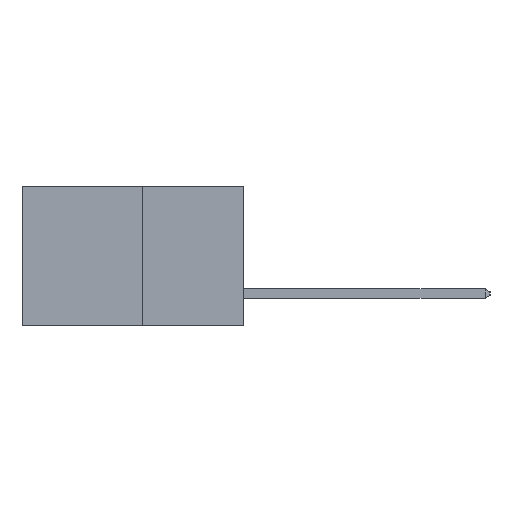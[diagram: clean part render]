
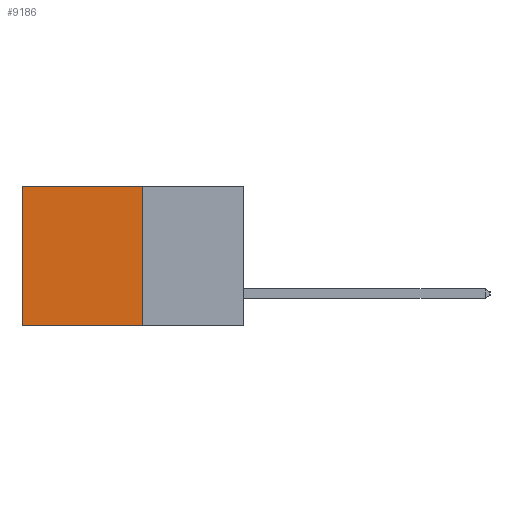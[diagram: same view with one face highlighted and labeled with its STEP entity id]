
A CAD part, left-side view. The second image highlights one B-rep face of the part: STEP entity #9186.
In plain terms, the highlighted planar face has unit normal (-1, 0, 0).
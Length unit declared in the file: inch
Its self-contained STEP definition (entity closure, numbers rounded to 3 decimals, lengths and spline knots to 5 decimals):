
#305 = VERTEX_POINT ( 'NONE', #18248 ) ;
#1296 = EDGE_CURVE ( 'NONE', #305, #4624, #8270, .T. ) ;
#1407 = CARTESIAN_POINT ( 'NONE',  ( 0.277, 0.59, 0. ) ) ;
#1757 = CARTESIAN_POINT ( 'NONE',  ( 0.277, 0.27, -0.37 ) ) ;
#2192 = VERTEX_POINT ( 'NONE', #10133 ) ;
#2246 = LINE ( 'NONE', #13829, #7796 ) ;
#2468 = ORIENTED_EDGE ( 'NONE', *, *, #18503, .F. ) ;
#3327 = VECTOR ( 'NONE', #10431, 39.37008 ) ;
#4147 = PLANE ( 'NONE',  #10761 ) ;
#4608 = EDGE_CURVE ( 'NONE', #4624, #13963, #8369, .T. ) ;
#4624 = VERTEX_POINT ( 'NONE', #1407 ) ;
#4732 = VECTOR ( 'NONE', #11727, 39.37008 ) ;
#5389 = FACE_OUTER_BOUND ( 'NONE', #13304, .T. ) ;
#6354 = CARTESIAN_POINT ( 'NONE',  ( 0.277, 0.59, -0.37 ) ) ;
#7559 = DIRECTION ( 'NONE',  ( 1., 0., 0. ) ) ;
#7796 = VECTOR ( 'NONE', #18578, 39.37008 ) ;
#8166 = LINE ( 'NONE', #1757, #4732 ) ;
#8270 = LINE ( 'NONE', #13934, #20627 ) ;
#8369 = LINE ( 'NONE', #6354, #3327 ) ;
#9186 = ADVANCED_FACE ( 'NONE', ( #5389 ), #4147, .F. ) ;
#10133 = CARTESIAN_POINT ( 'NONE',  ( 0.277, 0.27, -0.37 ) ) ;
#10417 = CARTESIAN_POINT ( 'NONE',  ( 0.277, 0.59, -0.37 ) ) ;
#10431 = DIRECTION ( 'NONE',  ( 0., 0., -1. ) ) ;
#10761 = AXIS2_PLACEMENT_3D ( 'NONE', #17292, #7559, #18899 ) ;
#11453 = ORIENTED_EDGE ( 'NONE', *, *, #13149, .F. ) ;
#11621 = ORIENTED_EDGE ( 'NONE', *, *, #1296, .T. ) ;
#11727 = DIRECTION ( 'NONE',  ( 0., 1., 0. ) ) ;
#11925 = DIRECTION ( 'NONE',  ( 0., 1., 0. ) ) ;
#13149 = EDGE_CURVE ( 'NONE', #2192, #13963, #8166, .T. ) ;
#13304 = EDGE_LOOP ( 'NONE', ( #17379, #11453, #2468, #11621 ) ) ;
#13829 = CARTESIAN_POINT ( 'NONE',  ( 0.277, 0.27, -0.37 ) ) ;
#13934 = CARTESIAN_POINT ( 'NONE',  ( 0.277, 0.27, 0. ) ) ;
#13963 = VERTEX_POINT ( 'NONE', #10417 ) ;
#17292 = CARTESIAN_POINT ( 'NONE',  ( 0.277, 0.27, -0.37 ) ) ;
#17379 = ORIENTED_EDGE ( 'NONE', *, *, #4608, .T. ) ;
#18248 = CARTESIAN_POINT ( 'NONE',  ( 0.277, 0.27, 0. ) ) ;
#18503 = EDGE_CURVE ( 'NONE', #305, #2192, #2246, .T. ) ;
#18578 = DIRECTION ( 'NONE',  ( 0., 0., -1. ) ) ;
#18899 = DIRECTION ( 'NONE',  ( 0., 0., -1. ) ) ;
#20627 = VECTOR ( 'NONE', #11925, 39.37008 ) ;
